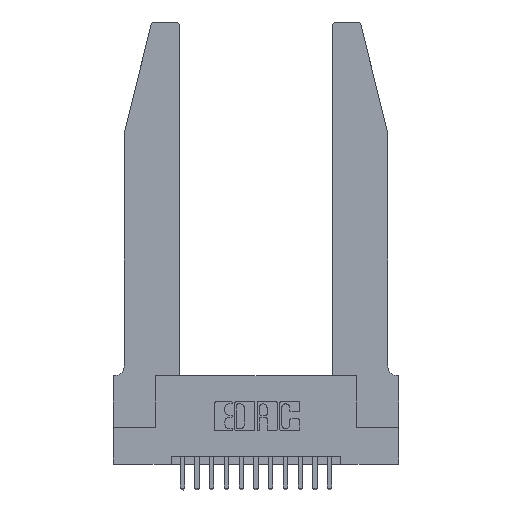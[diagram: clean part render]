
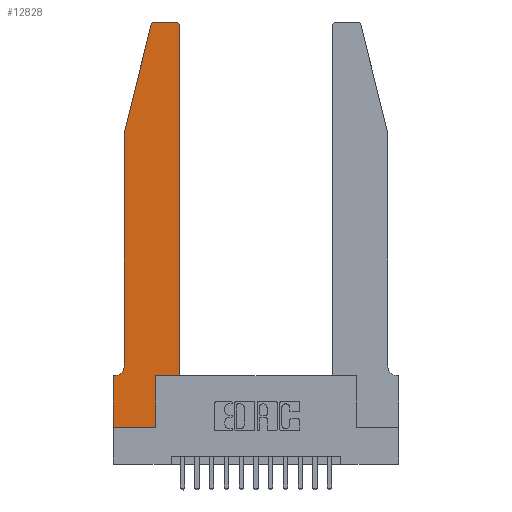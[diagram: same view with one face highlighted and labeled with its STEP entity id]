
A CAD part, top view. The second image highlights one B-rep face of the part: STEP entity #12828.
In plain terms, the highlighted planar face has unit normal (0, 0, 1).
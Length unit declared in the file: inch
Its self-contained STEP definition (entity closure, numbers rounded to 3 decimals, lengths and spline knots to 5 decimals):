
#63 = AXIS2_PLACEMENT_3D ( 'NONE', #7499, #921, #13214 ) ;
#109 = CIRCLE ( 'NONE', #8381, 0.03 ) ;
#128 = CARTESIAN_POINT ( 'NONE',  ( 0.0755, 2., 0.37 ) ) ;
#155 = VERTEX_POINT ( 'NONE', #3133 ) ;
#479 = EDGE_LOOP ( 'NONE', ( #7525, #1742, #16795, #7105, #7754, #4549, #15763, #6721, #14706, #2887, #7928, #17077 ) ) ;
#581 = DIRECTION ( 'NONE',  ( 1., 0., 0. ) ) ;
#675 = CIRCLE ( 'NONE', #10930, 0.03 ) ;
#706 = CARTESIAN_POINT ( 'NONE',  ( 0.4505, 0.35, 0.37 ) ) ;
#775 = EDGE_CURVE ( 'NONE', #6149, #6526, #7042, .T. ) ;
#921 = DIRECTION ( 'NONE',  ( 0., 0., -1. ) ) ;
#930 = CARTESIAN_POINT ( 'NONE',  ( 0.2865, 0.35, 0.37 ) ) ;
#1049 = EDGE_CURVE ( 'NONE', #10287, #155, #3801, .T. ) ;
#1293 = VECTOR ( 'NONE', #17022, 39.37008 ) ;
#1631 = LINE ( 'NONE', #11010, #5706 ) ;
#1742 = ORIENTED_EDGE ( 'NONE', *, *, #11351, .T. ) ;
#1819 = CARTESIAN_POINT ( 'NONE',  ( 0.284, 2.72, 0.37 ) ) ;
#2121 = LINE ( 'NONE', #4744, #1293 ) ;
#2544 = VECTOR ( 'NONE', #8062, 39.37008 ) ;
#2548 = PLANE ( 'NONE',  #12684 ) ;
#2718 = VECTOR ( 'NONE', #5980, 39.37008 ) ;
#2887 = ORIENTED_EDGE ( 'NONE', *, *, #12033, .T. ) ;
#3133 = CARTESIAN_POINT ( 'NONE',  ( 0.284, 2.75, 0.37 ) ) ;
#3137 = VECTOR ( 'NONE', #4082, 39.37008 ) ;
#3173 = DIRECTION ( 'NONE',  ( 0., 0., 1. ) ) ;
#3801 = LINE ( 'NONE', #17640, #3137 ) ;
#3813 = VERTEX_POINT ( 'NONE', #6770 ) ;
#3941 = CIRCLE ( 'NONE', #63, 0.07 ) ;
#4082 = DIRECTION ( 'NONE',  ( -1., 0., 0. ) ) ;
#4251 = VECTOR ( 'NONE', #17242, 39.37008 ) ;
#4283 = EDGE_CURVE ( 'NONE', #3813, #12578, #8837, .T. ) ;
#4305 = CARTESIAN_POINT ( 'NONE',  ( 0.0755, 2., 0.37 ) ) ;
#4484 = VERTEX_POINT ( 'NONE', #5152 ) ;
#4549 = ORIENTED_EDGE ( 'NONE', *, *, #14670, .T. ) ;
#4744 = CARTESIAN_POINT ( 'NONE',  ( 0.4505, 0.35, 0.37 ) ) ;
#5152 = CARTESIAN_POINT ( 'NONE',  ( 0.4505, 2.72, 0.37 ) ) ;
#5265 = DIRECTION ( 'NONE',  ( 0., 0., 1. ) ) ;
#5392 = VERTEX_POINT ( 'NONE', #7681 ) ;
#5706 = VECTOR ( 'NONE', #16271, 39.37008 ) ;
#5840 = VECTOR ( 'NONE', #13117, 39.37008 ) ;
#5980 = DIRECTION ( 'NONE',  ( 0., 1., 0. ) ) ;
#6051 = EDGE_CURVE ( 'NONE', #11176, #4484, #2121, .T. ) ;
#6149 = VERTEX_POINT ( 'NONE', #15440 ) ;
#6190 = LINE ( 'NONE', #14825, #2544 ) ;
#6261 = CARTESIAN_POINT ( 'NONE',  ( 0., 0., 0.37 ) ) ;
#6526 = VERTEX_POINT ( 'NONE', #930 ) ;
#6721 = ORIENTED_EDGE ( 'NONE', *, *, #12062, .T. ) ;
#6770 = CARTESIAN_POINT ( 'NONE',  ( 0.25487, 2.72718, 0.37 ) ) ;
#7001 = DIRECTION ( 'NONE',  ( 1., 0., 0. ) ) ;
#7042 = LINE ( 'NONE', #7198, #2718 ) ;
#7105 = ORIENTED_EDGE ( 'NONE', *, *, #12142, .T. ) ;
#7198 = CARTESIAN_POINT ( 'NONE',  ( 0.2865, 0.35, 0.37 ) ) ;
#7465 = EDGE_CURVE ( 'NONE', #12849, #8193, #7876, .T. ) ;
#7499 = CARTESIAN_POINT ( 'NONE',  ( 0.0055, 0.42, 0.37 ) ) ;
#7525 = ORIENTED_EDGE ( 'NONE', *, *, #1049, .T. ) ;
#7681 = CARTESIAN_POINT ( 'NONE',  ( 0.0055, 0.35, 0.37 ) ) ;
#7754 = ORIENTED_EDGE ( 'NONE', *, *, #10089, .T. ) ;
#7876 = LINE ( 'NONE', #6261, #4251 ) ;
#7928 = ORIENTED_EDGE ( 'NONE', *, *, #6051, .T. ) ;
#8062 = DIRECTION ( 'NONE',  ( 1., 0., 0. ) ) ;
#8193 = VERTEX_POINT ( 'NONE', #10889 ) ;
#8381 = AXIS2_PLACEMENT_3D ( 'NONE', #15256, #12532, #7001 ) ;
#8763 = FACE_OUTER_BOUND ( 'NONE', #479, .T. ) ;
#8837 = LINE ( 'NONE', #10480, #5840 ) ;
#9234 = CARTESIAN_POINT ( 'NONE',  ( 0.0755, 0.42, 0.37 ) ) ;
#10089 = EDGE_CURVE ( 'NONE', #15185, #5392, #3941, .T. ) ;
#10287 = VERTEX_POINT ( 'NONE', #15892 ) ;
#10480 = CARTESIAN_POINT ( 'NONE',  ( 0.0755, 2., 0.37 ) ) ;
#10794 = CARTESIAN_POINT ( 'NONE',  ( 0., 0.35, 0.37 ) ) ;
#10889 = CARTESIAN_POINT ( 'NONE',  ( 0., 0., 0.37 ) ) ;
#10930 = AXIS2_PLACEMENT_3D ( 'NONE', #1819, #3173, #581 ) ;
#11010 = CARTESIAN_POINT ( 'NONE',  ( 0.0755, 0.35, 0.37 ) ) ;
#11176 = VERTEX_POINT ( 'NONE', #13049 ) ;
#11351 = EDGE_CURVE ( 'NONE', #155, #3813, #675, .T. ) ;
#12033 = EDGE_CURVE ( 'NONE', #6526, #11176, #14317, .T. ) ;
#12062 = EDGE_CURVE ( 'NONE', #8193, #6149, #6190, .T. ) ;
#12142 = EDGE_CURVE ( 'NONE', #12578, #15185, #15195, .T. ) ;
#12374 = VECTOR ( 'NONE', #13905, 39.37008 ) ;
#12532 = DIRECTION ( 'NONE',  ( 0., 0., 1. ) ) ;
#12578 = VERTEX_POINT ( 'NONE', #128 ) ;
#12684 = AXIS2_PLACEMENT_3D ( 'NONE', #10794, #5265, #13497 ) ;
#12828 = ADVANCED_FACE ( 'NONE', ( #8763 ), #2548, .T. ) ;
#12849 = VERTEX_POINT ( 'NONE', #13437 ) ;
#13049 = CARTESIAN_POINT ( 'NONE',  ( 0.4505, 0.35, 0.37 ) ) ;
#13117 = DIRECTION ( 'NONE',  ( -0.239, -0.971, 0. ) ) ;
#13214 = DIRECTION ( 'NONE',  ( -1., 0., 0. ) ) ;
#13437 = CARTESIAN_POINT ( 'NONE',  ( 0., 0.35, 0.37 ) ) ;
#13497 = DIRECTION ( 'NONE',  ( 1., 0., 0. ) ) ;
#13905 = DIRECTION ( 'NONE',  ( 0., -1., 0. ) ) ;
#14317 = LINE ( 'NONE', #706, #17082 ) ;
#14518 = DIRECTION ( 'NONE',  ( 1., 0., 0. ) ) ;
#14670 = EDGE_CURVE ( 'NONE', #5392, #12849, #1631, .T. ) ;
#14706 = ORIENTED_EDGE ( 'NONE', *, *, #775, .T. ) ;
#14825 = CARTESIAN_POINT ( 'NONE',  ( 0., 0., 0.37 ) ) ;
#15185 = VERTEX_POINT ( 'NONE', #9234 ) ;
#15195 = LINE ( 'NONE', #4305, #12374 ) ;
#15256 = CARTESIAN_POINT ( 'NONE',  ( 0.4205, 2.72, 0.37 ) ) ;
#15440 = CARTESIAN_POINT ( 'NONE',  ( 0.2865, 0., 0.37 ) ) ;
#15763 = ORIENTED_EDGE ( 'NONE', *, *, #7465, .T. ) ;
#15869 = EDGE_CURVE ( 'NONE', #4484, #10287, #109, .T. ) ;
#15892 = CARTESIAN_POINT ( 'NONE',  ( 0.4205, 2.75, 0.37 ) ) ;
#16271 = DIRECTION ( 'NONE',  ( -1., 0., 0. ) ) ;
#16795 = ORIENTED_EDGE ( 'NONE', *, *, #4283, .T. ) ;
#17022 = DIRECTION ( 'NONE',  ( 0., 1., 0. ) ) ;
#17077 = ORIENTED_EDGE ( 'NONE', *, *, #15869, .T. ) ;
#17082 = VECTOR ( 'NONE', #14518, 39.37008 ) ;
#17242 = DIRECTION ( 'NONE',  ( 0., -1., 0. ) ) ;
#17640 = CARTESIAN_POINT ( 'NONE',  ( 0.2605, 2.75, 0.37 ) ) ;
